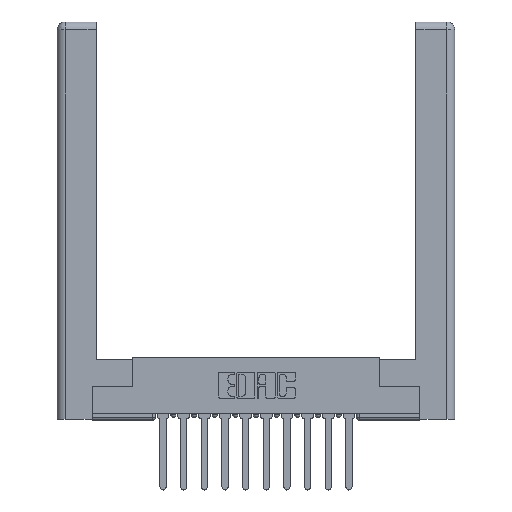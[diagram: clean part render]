
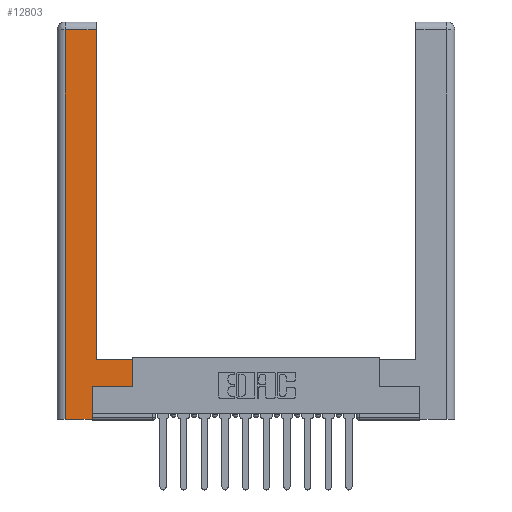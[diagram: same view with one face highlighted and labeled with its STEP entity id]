
A CAD part, top view. The second image highlights one B-rep face of the part: STEP entity #12803.
In plain terms, the highlighted planar face has unit normal (0, 0, 1).
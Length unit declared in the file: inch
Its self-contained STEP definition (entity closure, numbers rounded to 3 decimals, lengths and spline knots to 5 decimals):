
#76 = CARTESIAN_POINT ( 'NONE',  ( 0.565, 0.45, 0. ) ) ;
#127 = LINE ( 'NONE', #13042, #3617 ) ;
#584 = VERTEX_POINT ( 'NONE', #687 ) ;
#687 = CARTESIAN_POINT ( 'NONE',  ( 0.565, 0.45, 0. ) ) ;
#987 = EDGE_CURVE ( 'NONE', #13525, #12838, #1362, .T. ) ;
#1334 = DIRECTION ( 'NONE',  ( 1., 0., 0. ) ) ;
#1362 = LINE ( 'NONE', #6054, #1476 ) ;
#1476 = VECTOR ( 'NONE', #2372, 39.37008 ) ;
#1527 = DIRECTION ( 'NONE',  ( 0., 1., 0. ) ) ;
#1749 = AXIS2_PLACEMENT_3D ( 'NONE', #7738, #8666, #1838 ) ;
#1802 = CARTESIAN_POINT ( 'NONE',  ( 0.265, 0., 0. ) ) ;
#1838 = DIRECTION ( 'NONE',  ( -1., 0., 0. ) ) ;
#2237 = EDGE_CURVE ( 'NONE', #14476, #584, #3692, .T. ) ;
#2243 = DIRECTION ( 'NONE',  ( -1., 0., 0. ) ) ;
#2372 = DIRECTION ( 'NONE',  ( 0., 1., 0. ) ) ;
#2514 = ORIENTED_EDGE ( 'NONE', *, *, #2237, .T. ) ;
#3068 = PLANE ( 'NONE',  #1749 ) ;
#3553 = CARTESIAN_POINT ( 'NONE',  ( 0.295, 0.45, 0. ) ) ;
#3617 = VECTOR ( 'NONE', #12965, 39.37008 ) ;
#3692 = LINE ( 'NONE', #76, #11829 ) ;
#3734 = CARTESIAN_POINT ( 'NONE',  ( 0.565, 0.245, 0. ) ) ;
#4132 = VERTEX_POINT ( 'NONE', #7791 ) ;
#4346 = CARTESIAN_POINT ( 'NONE',  ( 0.0615, 2.94, 0. ) ) ;
#4568 = DIRECTION ( 'NONE',  ( 0., 1., 0. ) ) ;
#4593 = VECTOR ( 'NONE', #1334, 39.37008 ) ;
#5178 = EDGE_CURVE ( 'NONE', #13423, #14476, #9455, .T. ) ;
#5526 = EDGE_CURVE ( 'NONE', #4132, #5771, #7917, .T. ) ;
#5541 = EDGE_CURVE ( 'NONE', #584, #13525, #10744, .T. ) ;
#5573 = CARTESIAN_POINT ( 'NONE',  ( 0.265, 0.245, 0. ) ) ;
#5771 = VERTEX_POINT ( 'NONE', #11955 ) ;
#6054 = CARTESIAN_POINT ( 'NONE',  ( 0.295, 3., 0. ) ) ;
#6072 = VECTOR ( 'NONE', #8013, 39.37008 ) ;
#6252 = EDGE_CURVE ( 'NONE', #12838, #4132, #8090, .T. ) ;
#6965 = ORIENTED_EDGE ( 'NONE', *, *, #5178, .T. ) ;
#6977 = ORIENTED_EDGE ( 'NONE', *, *, #14779, .T. ) ;
#7136 = ORIENTED_EDGE ( 'NONE', *, *, #987, .T. ) ;
#7257 = CARTESIAN_POINT ( 'NONE',  ( 0.565, 0.245, 0. ) ) ;
#7738 = CARTESIAN_POINT ( 'NONE',  ( 0., 0., 0. ) ) ;
#7791 = CARTESIAN_POINT ( 'NONE',  ( 0.0615, 2.94, 0. ) ) ;
#7806 = ORIENTED_EDGE ( 'NONE', *, *, #6252, .T. ) ;
#7819 = CARTESIAN_POINT ( 'NONE',  ( 0.295, 2.94, 0. ) ) ;
#7874 = LINE ( 'NONE', #13899, #10279 ) ;
#7917 = LINE ( 'NONE', #12556, #10636 ) ;
#8013 = DIRECTION ( 'NONE',  ( -1., 0., 0. ) ) ;
#8090 = LINE ( 'NONE', #4346, #6072 ) ;
#8185 = VECTOR ( 'NONE', #2243, 39.37008 ) ;
#8666 = DIRECTION ( 'NONE',  ( 0., 0., -1. ) ) ;
#8962 = FACE_OUTER_BOUND ( 'NONE', #15033, .T. ) ;
#9455 = LINE ( 'NONE', #3734, #4593 ) ;
#9633 = EDGE_CURVE ( 'NONE', #5771, #12745, #127, .T. ) ;
#10279 = VECTOR ( 'NONE', #4568, 39.37008 ) ;
#10630 = ORIENTED_EDGE ( 'NONE', *, *, #5541, .T. ) ;
#10636 = VECTOR ( 'NONE', #12935, 39.37008 ) ;
#10744 = LINE ( 'NONE', #3553, #8185 ) ;
#11829 = VECTOR ( 'NONE', #1527, 39.37008 ) ;
#11955 = CARTESIAN_POINT ( 'NONE',  ( 0.0615, 0., 0. ) ) ;
#12556 = CARTESIAN_POINT ( 'NONE',  ( 0.0615, 0., 0. ) ) ;
#12745 = VERTEX_POINT ( 'NONE', #1802 ) ;
#12803 = ADVANCED_FACE ( 'NONE', ( #8962 ), #3068, .F. ) ;
#12838 = VERTEX_POINT ( 'NONE', #7819 ) ;
#12935 = DIRECTION ( 'NONE',  ( 0., -1., 0. ) ) ;
#12965 = DIRECTION ( 'NONE',  ( 1., 0., 0. ) ) ;
#13042 = CARTESIAN_POINT ( 'NONE',  ( 0.265, 0., 0. ) ) ;
#13114 = CARTESIAN_POINT ( 'NONE',  ( 0.295, 0.45, 0. ) ) ;
#13215 = ORIENTED_EDGE ( 'NONE', *, *, #9633, .T. ) ;
#13423 = VERTEX_POINT ( 'NONE', #5573 ) ;
#13525 = VERTEX_POINT ( 'NONE', #13114 ) ;
#13814 = ORIENTED_EDGE ( 'NONE', *, *, #5526, .T. ) ;
#13899 = CARTESIAN_POINT ( 'NONE',  ( 0.265, 0.245, 0. ) ) ;
#14476 = VERTEX_POINT ( 'NONE', #7257 ) ;
#14779 = EDGE_CURVE ( 'NONE', #12745, #13423, #7874, .T. ) ;
#15033 = EDGE_LOOP ( 'NONE', ( #7136, #7806, #13814, #13215, #6977, #6965, #2514, #10630 ) ) ;
